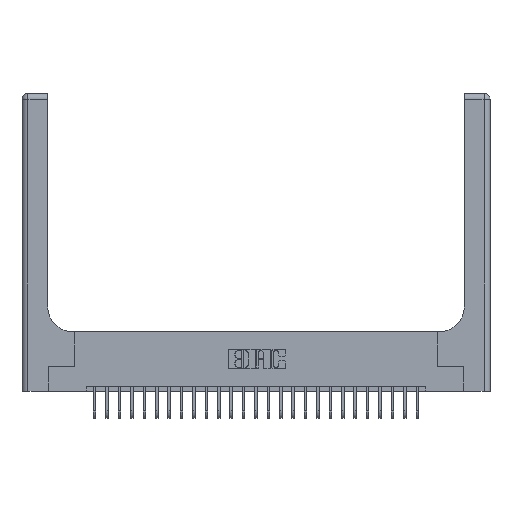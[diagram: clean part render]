
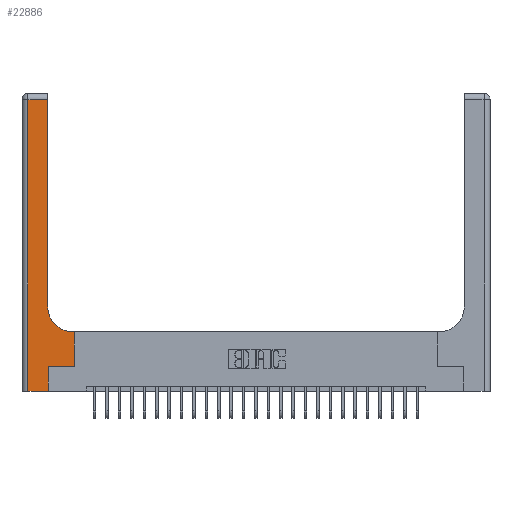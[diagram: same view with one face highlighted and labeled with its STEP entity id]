
A CAD part, top view. The second image highlights one B-rep face of the part: STEP entity #22886.
In plain terms, the highlighted planar face has unit normal (0, 0, 1).
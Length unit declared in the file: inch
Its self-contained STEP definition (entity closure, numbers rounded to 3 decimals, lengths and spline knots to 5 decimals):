
#971 = VECTOR ( 'NONE', #1902, 39.37008 ) ;
#1080 = CARTESIAN_POINT ( 'NONE',  ( 0.26, 0.85, 0.37 ) ) ;
#1553 = VECTOR ( 'NONE', #20085, 39.37008 ) ;
#1902 = DIRECTION ( 'NONE',  ( 0., 1., 0. ) ) ;
#2202 = DIRECTION ( 'NONE',  ( 0., 1., 0. ) ) ;
#2755 = VERTEX_POINT ( 'NONE', #1080 ) ;
#3054 = EDGE_CURVE ( 'NONE', #15597, #11929, #20710, .T. ) ;
#3127 = LINE ( 'NONE', #12508, #21086 ) ;
#3137 = VERTEX_POINT ( 'NONE', #13375 ) ;
#3999 = CARTESIAN_POINT ( 'NONE',  ( 0., 2.94, 0.37 ) ) ;
#4217 = EDGE_CURVE ( 'NONE', #13673, #13691, #21516, .T. ) ;
#4386 = VERTEX_POINT ( 'NONE', #7742 ) ;
#4818 = FACE_OUTER_BOUND ( 'NONE', #19851, .T. ) ;
#5302 = CARTESIAN_POINT ( 'NONE',  ( 0.528, 0.25, 0.37 ) ) ;
#5706 = CARTESIAN_POINT ( 'NONE',  ( 0.265, 0., 0.37 ) ) ;
#6413 = DIRECTION ( 'NONE',  ( -1., 0., 0. ) ) ;
#6528 = LINE ( 'NONE', #17814, #20641 ) ;
#6559 = DIRECTION ( 'NONE',  ( 0., 0., -1. ) ) ;
#7348 = DIRECTION ( 'NONE',  ( 0., -1., 0. ) ) ;
#7614 = EDGE_CURVE ( 'NONE', #11929, #10600, #6528, .T. ) ;
#7742 = CARTESIAN_POINT ( 'NONE',  ( 0.06, 0., 0.37 ) ) ;
#7895 = ORIENTED_EDGE ( 'NONE', *, *, #11174, .T. ) ;
#8226 = CARTESIAN_POINT ( 'NONE',  ( 0., 3., 0.37 ) ) ;
#9136 = ORIENTED_EDGE ( 'NONE', *, *, #15303, .T. ) ;
#9466 = CIRCLE ( 'NONE', #15022, 0.25 ) ;
#9936 = VECTOR ( 'NONE', #15735, 39.37008 ) ;
#10066 = CARTESIAN_POINT ( 'NONE',  ( 0.265, 0.25, 0.37 ) ) ;
#10600 = VERTEX_POINT ( 'NONE', #5302 ) ;
#10630 = VERTEX_POINT ( 'NONE', #12822 ) ;
#10759 = ORIENTED_EDGE ( 'NONE', *, *, #7614, .T. ) ;
#11174 = EDGE_CURVE ( 'NONE', #13691, #4386, #21726, .T. ) ;
#11739 = EDGE_CURVE ( 'NONE', #4386, #15597, #21263, .T. ) ;
#11929 = VERTEX_POINT ( 'NONE', #10066 ) ;
#12014 = VECTOR ( 'NONE', #7348, 39.37008 ) ;
#12508 = CARTESIAN_POINT ( 'NONE',  ( 0.26, 3., 0.37 ) ) ;
#12822 = CARTESIAN_POINT ( 'NONE',  ( 0.528, 0.6, 0.37 ) ) ;
#12937 = ORIENTED_EDGE ( 'NONE', *, *, #13043, .T. ) ;
#13043 = EDGE_CURVE ( 'NONE', #3137, #2755, #9466, .T. ) ;
#13375 = CARTESIAN_POINT ( 'NONE',  ( 0.51, 0.6, 0.37 ) ) ;
#13673 = VERTEX_POINT ( 'NONE', #17765 ) ;
#13691 = VERTEX_POINT ( 'NONE', #23410 ) ;
#14336 = ORIENTED_EDGE ( 'NONE', *, *, #3054, .T. ) ;
#14709 = EDGE_CURVE ( 'NONE', #10630, #3137, #14860, .T. ) ;
#14860 = LINE ( 'NONE', #22967, #9936 ) ;
#15022 = AXIS2_PLACEMENT_3D ( 'NONE', #17625, #6559, #19449 ) ;
#15303 = EDGE_CURVE ( 'NONE', #2755, #13673, #3127, .T. ) ;
#15350 = CARTESIAN_POINT ( 'NONE',  ( 0.528, 0.25, 0.37 ) ) ;
#15597 = VERTEX_POINT ( 'NONE', #20781 ) ;
#15659 = PLANE ( 'NONE',  #21006 ) ;
#15735 = DIRECTION ( 'NONE',  ( -1., 0., 0. ) ) ;
#16238 = EDGE_CURVE ( 'NONE', #10600, #10630, #20787, .T. ) ;
#16468 = CARTESIAN_POINT ( 'NONE',  ( 0.06, 3., 0.37 ) ) ;
#17003 = DIRECTION ( 'NONE',  ( -1., 0., 0. ) ) ;
#17490 = DIRECTION ( 'NONE',  ( 0., 0., -1. ) ) ;
#17625 = CARTESIAN_POINT ( 'NONE',  ( 0.51, 0.85, 0.37 ) ) ;
#17765 = CARTESIAN_POINT ( 'NONE',  ( 0.26, 2.94, 0.37 ) ) ;
#17814 = CARTESIAN_POINT ( 'NONE',  ( 0.265, 0.25, 0.37 ) ) ;
#18259 = CARTESIAN_POINT ( 'NONE',  ( 0., 0., 0.37 ) ) ;
#18389 = ORIENTED_EDGE ( 'NONE', *, *, #4217, .T. ) ;
#19449 = DIRECTION ( 'NONE',  ( 1., 0., 0. ) ) ;
#19628 = DIRECTION ( 'NONE',  ( 1., 0., 0. ) ) ;
#19851 = EDGE_LOOP ( 'NONE', ( #9136, #18389, #7895, #23210, #14336, #10759, #23898, #21821, #12937 ) ) ;
#20085 = DIRECTION ( 'NONE',  ( 1., 0., 0. ) ) ;
#20211 = VECTOR ( 'NONE', #2202, 39.37008 ) ;
#20641 = VECTOR ( 'NONE', #19628, 39.37008 ) ;
#20710 = LINE ( 'NONE', #5706, #971 ) ;
#20781 = CARTESIAN_POINT ( 'NONE',  ( 0.265, 0., 0.37 ) ) ;
#20787 = LINE ( 'NONE', #15350, #20211 ) ;
#21006 = AXIS2_PLACEMENT_3D ( 'NONE', #8226, #17490, #6413 ) ;
#21086 = VECTOR ( 'NONE', #21573, 39.37008 ) ;
#21263 = LINE ( 'NONE', #18259, #1553 ) ;
#21516 = LINE ( 'NONE', #3999, #22094 ) ;
#21573 = DIRECTION ( 'NONE',  ( 0., 1., 0. ) ) ;
#21726 = LINE ( 'NONE', #16468, #12014 ) ;
#21821 = ORIENTED_EDGE ( 'NONE', *, *, #14709, .T. ) ;
#22094 = VECTOR ( 'NONE', #17003, 39.37008 ) ;
#22886 = ADVANCED_FACE ( 'NONE', ( #4818 ), #15659, .F. ) ;
#22967 = CARTESIAN_POINT ( 'NONE',  ( 0.26, 0.6, 0.37 ) ) ;
#23210 = ORIENTED_EDGE ( 'NONE', *, *, #11739, .T. ) ;
#23410 = CARTESIAN_POINT ( 'NONE',  ( 0.06, 2.94, 0.37 ) ) ;
#23898 = ORIENTED_EDGE ( 'NONE', *, *, #16238, .T. ) ;
